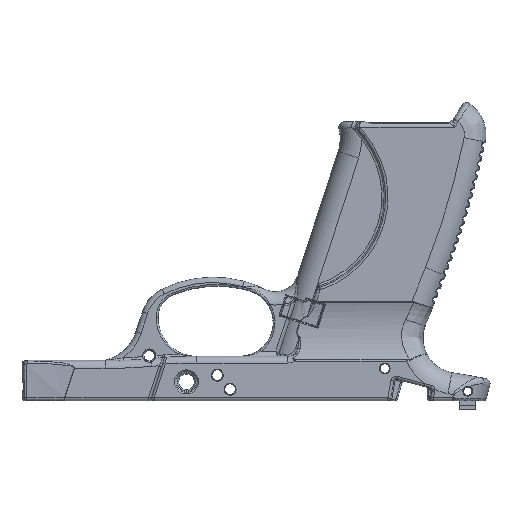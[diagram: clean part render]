
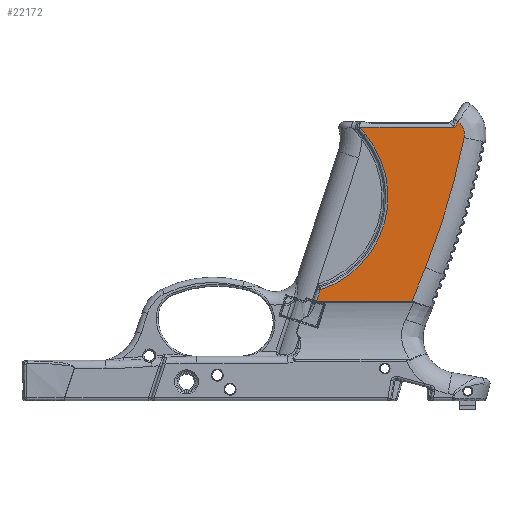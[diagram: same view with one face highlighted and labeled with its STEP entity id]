
A CAD part, front view. The second image highlights one B-rep face of the part: STEP entity #22172.
In plain terms, the highlighted planar face has unit normal (0, -1, 0).
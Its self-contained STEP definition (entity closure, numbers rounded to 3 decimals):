
#1113=PLANE('',#24168);
#1815=FACE_OUTER_BOUND('',#3317,.T.);
#3317=EDGE_LOOP('',(#16927,#16928,#16929,#16930,#16931,#16932,#16933,#16934,
#16935,#16936,#16937));
#4534=CIRCLE('',#23632,282.274);
#4808=CIRCLE('',#24169,6.);
#4809=CIRCLE('',#24170,36.518);
#6029=LINE('',#43325,#7118);
#6211=LINE('',#47040,#7300);
#6214=LINE('',#47063,#7303);
#6215=LINE('',#47066,#7304);
#6216=LINE('',#47070,#7305);
#6217=LINE('',#47072,#7306);
#7118=VECTOR('',#27441,10.);
#7300=VECTOR('',#28403,10.);
#7303=VECTOR('',#28416,10.);
#7304=VECTOR('',#28421,10.);
#7305=VECTOR('',#28424,10.);
#7306=VECTOR('',#28425,10.);
#8189=B_SPLINE_CURVE_WITH_KNOTS('',3,(#47074,#47075,#47076,#47077),
 .UNSPECIFIED.,.F.,.F.,(4,4),(0.,0.042),
 .UNSPECIFIED.);
#8190=B_SPLINE_CURVE_WITH_KNOTS('',3,(#47079,#47080,#47081,#47082),
 .UNSPECIFIED.,.F.,.F.,(4,4),(-0.882,-0.597),
 .UNSPECIFIED.);
#9116=VERTEX_POINT('',#38317);
#9117=VERTEX_POINT('',#38319);
#9230=VERTEX_POINT('',#43324);
#9555=VERTEX_POINT('',#46990);
#9556=VERTEX_POINT('',#47013);
#9562=VERTEX_POINT('',#47062);
#9563=VERTEX_POINT('',#47067);
#9564=VERTEX_POINT('',#47069);
#9565=VERTEX_POINT('',#47071);
#9566=VERTEX_POINT('',#47073);
#9567=VERTEX_POINT('',#47078);
#11367=EDGE_CURVE('',#9116,#9117,#4534,.T.);
#11591=EDGE_CURVE('',#9117,#9230,#6029,.T.);
#12132=EDGE_CURVE('',#9556,#9555,#6211,.T.);
#12139=EDGE_CURVE('',#9555,#9562,#6214,.T.);
#12141=EDGE_CURVE('',#9230,#9556,#6215,.T.);
#12142=EDGE_CURVE('',#9563,#9116,#4808,.T.);
#12143=EDGE_CURVE('',#9564,#9563,#6216,.T.);
#12144=EDGE_CURVE('',#9565,#9564,#6217,.T.);
#12145=EDGE_CURVE('',#9566,#9565,#8189,.T.);
#12146=EDGE_CURVE('',#9567,#9566,#8190,.T.);
#12147=EDGE_CURVE('',#9562,#9567,#4809,.T.);
#16927=ORIENTED_EDGE('',*,*,#12132,.F.);
#16928=ORIENTED_EDGE('',*,*,#12141,.F.);
#16929=ORIENTED_EDGE('',*,*,#11591,.F.);
#16930=ORIENTED_EDGE('',*,*,#11367,.F.);
#16931=ORIENTED_EDGE('',*,*,#12142,.F.);
#16932=ORIENTED_EDGE('',*,*,#12143,.F.);
#16933=ORIENTED_EDGE('',*,*,#12144,.F.);
#16934=ORIENTED_EDGE('',*,*,#12145,.F.);
#16935=ORIENTED_EDGE('',*,*,#12146,.F.);
#16936=ORIENTED_EDGE('',*,*,#12147,.F.);
#16937=ORIENTED_EDGE('',*,*,#12139,.F.);
#22172=ADVANCED_FACE('',(#1815),#1113,.T.);
#23632=AXIS2_PLACEMENT_3D('',#38320,#27101,#27102);
#24168=AXIS2_PLACEMENT_3D('',#47065,#28419,#28420);
#24169=AXIS2_PLACEMENT_3D('',#47068,#28422,#28423);
#24170=AXIS2_PLACEMENT_3D('',#47083,#28426,#28427);
#27101=DIRECTION('center_axis',(0.,1.,0.));
#27102=DIRECTION('ref_axis',(0.958,0.,-0.286));
#27441=DIRECTION('',(-0.371,0.,-0.929));
#28403=DIRECTION('',(-0.952,0.,0.306));
#28416=DIRECTION('',(0.309,0.,0.951));
#28419=DIRECTION('center_axis',(0.,-1.,0.));
#28420=DIRECTION('ref_axis',(1.,0.,0.));
#28421=DIRECTION('',(-1.,0.,0.));
#28422=DIRECTION('center_axis',(0.,1.,0.));
#28423=DIRECTION('ref_axis',(0.863,0.,0.505));
#28424=DIRECTION('',(0.531,0.,0.848));
#28425=DIRECTION('',(1.,0.,0.));
#28426=DIRECTION('center_axis',(0.,-1.,0.));
#28427=DIRECTION('ref_axis',(0.962,0.,-0.272));
#38317=CARTESIAN_POINT('',(89.046,-13.75,58.092));
#38319=CARTESIAN_POINT('',(74.571,-13.75,9.633));
#38320=CARTESIAN_POINT('Origin',(-187.57,-13.75,114.326));
#43324=CARTESIAN_POINT('',(69.538,-13.75,-2.968));
#43325=CARTESIAN_POINT('',(77.289,-13.75,16.44));
#46990=CARTESIAN_POINT('',(33.966,-13.75,-2.917));
#47013=CARTESIAN_POINT('',(34.127,-13.75,-2.968));
#47040=CARTESIAN_POINT('',(39.085,-13.75,-4.56));
#47062=CARTESIAN_POINT('',(35.343,-13.75,1.321));
#47063=CARTESIAN_POINT('',(36.084,-13.75,3.6));
#47065=CARTESIAN_POINT('Origin',(62.214,-13.75,30.354));
#47066=CARTESIAN_POINT('',(110.,-13.75,-2.968));
#47067=CARTESIAN_POINT('',(86.781,-13.75,64.076));
#47068=CARTESIAN_POINT('Origin',(83.166,-13.75,59.287));
#47069=CARTESIAN_POINT('',(85.482,-13.75,62.));
#47070=CARTESIAN_POINT('',(75.697,-13.75,46.369));
#47071=CARTESIAN_POINT('',(50.085,-13.75,62.));
#47072=CARTESIAN_POINT('',(51.607,-13.75,62.));
#47073=CARTESIAN_POINT('',(50.244,-13.75,61.619));
#47074=CARTESIAN_POINT('Ctrl Pts',(50.244,-13.75,61.619));
#47075=CARTESIAN_POINT('Ctrl Pts',(50.149,-13.75,61.723));
#47076=CARTESIAN_POINT('Ctrl Pts',(50.085,-13.75,61.859));
#47077=CARTESIAN_POINT('Ctrl Pts',(50.085,-13.75,62.));
#47078=CARTESIAN_POINT('',(52.112,-13.75,59.473));
#47079=CARTESIAN_POINT('Ctrl Pts',(52.112,-13.75,59.473));
#47080=CARTESIAN_POINT('Ctrl Pts',(51.504,-13.75,60.201));
#47081=CARTESIAN_POINT('Ctrl Pts',(50.881,-13.75,60.916));
#47082=CARTESIAN_POINT('Ctrl Pts',(50.244,-13.75,61.619));
#47083=CARTESIAN_POINT('Origin',(24.087,-13.75,36.061));
